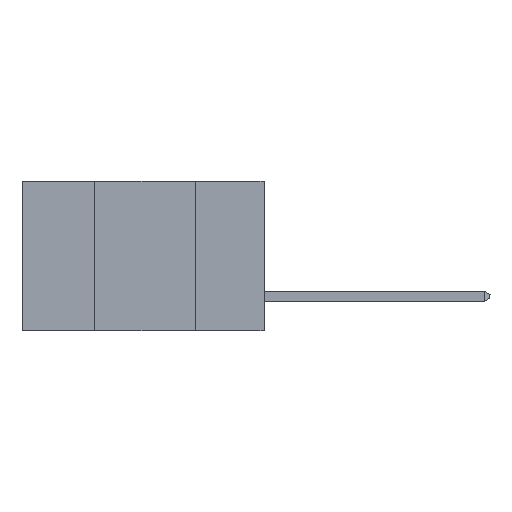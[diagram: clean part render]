
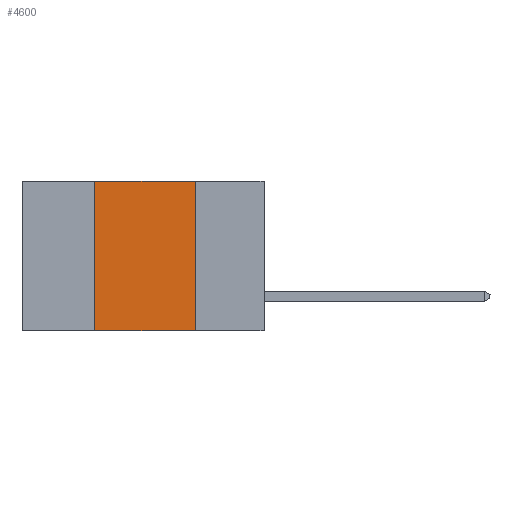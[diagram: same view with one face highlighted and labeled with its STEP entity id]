
A CAD part, left-side view. The second image highlights one B-rep face of the part: STEP entity #4600.
In plain terms, the highlighted planar face has unit normal (-1, 0, 0).
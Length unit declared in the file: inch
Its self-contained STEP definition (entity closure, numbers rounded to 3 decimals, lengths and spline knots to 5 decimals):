
#760 = VECTOR ( 'NONE', #7964, 39.37008 ) ;
#1302 = CARTESIAN_POINT ( 'NONE',  ( 0., 0.17, -0.37 ) ) ;
#1324 = ORIENTED_EDGE ( 'NONE', *, *, #4816, .F. ) ;
#1356 = CARTESIAN_POINT ( 'NONE',  ( 0., 0.6, 0. ) ) ;
#1605 = DIRECTION ( 'NONE',  ( 1., 0., 0. ) ) ;
#2115 = CARTESIAN_POINT ( 'NONE',  ( 0., 0.6, -0.37 ) ) ;
#2451 = LINE ( 'NONE', #1356, #6887 ) ;
#2771 = CARTESIAN_POINT ( 'NONE',  ( 0., 0.6, 0. ) ) ;
#3345 = VECTOR ( 'NONE', #13911, 39.37008 ) ;
#3355 = LINE ( 'NONE', #11182, #760 ) ;
#3362 = VERTEX_POINT ( 'NONE', #8556 ) ;
#3592 = PLANE ( 'NONE',  #10115 ) ;
#3668 = EDGE_CURVE ( 'NONE', #3362, #10784, #4863, .T. ) ;
#3770 = VERTEX_POINT ( 'NONE', #8732 ) ;
#4344 = EDGE_CURVE ( 'NONE', #6129, #10784, #7761, .T. ) ;
#4600 = ADVANCED_FACE ( 'NONE', ( #4975 ), #3592, .F. ) ;
#4816 = EDGE_CURVE ( 'NONE', #6129, #3770, #3355, .T. ) ;
#4863 = LINE ( 'NONE', #11534, #3345 ) ;
#4975 = FACE_OUTER_BOUND ( 'NONE', #6403, .T. ) ;
#5325 = ORIENTED_EDGE ( 'NONE', *, *, #3668, .F. ) ;
#6129 = VERTEX_POINT ( 'NONE', #7472 ) ;
#6403 = EDGE_LOOP ( 'NONE', ( #5325, #11475, #1324, #10087 ) ) ;
#6774 = EDGE_CURVE ( 'NONE', #3770, #3362, #2451, .T. ) ;
#6887 = VECTOR ( 'NONE', #13627, 39.37008 ) ;
#7472 = CARTESIAN_POINT ( 'NONE',  ( 0., 0.42, -0.37 ) ) ;
#7761 = LINE ( 'NONE', #2115, #8001 ) ;
#7964 = DIRECTION ( 'NONE',  ( 0., 0., 1. ) ) ;
#8001 = VECTOR ( 'NONE', #13445, 39.37008 ) ;
#8556 = CARTESIAN_POINT ( 'NONE',  ( 0., 0.17, 0. ) ) ;
#8732 = CARTESIAN_POINT ( 'NONE',  ( 0., 0.42, 0. ) ) ;
#10087 = ORIENTED_EDGE ( 'NONE', *, *, #4344, .T. ) ;
#10115 = AXIS2_PLACEMENT_3D ( 'NONE', #2771, #1605, #12685 ) ;
#10784 = VERTEX_POINT ( 'NONE', #1302 ) ;
#11182 = CARTESIAN_POINT ( 'NONE',  ( 0., 0.42, -0.37 ) ) ;
#11475 = ORIENTED_EDGE ( 'NONE', *, *, #6774, .F. ) ;
#11534 = CARTESIAN_POINT ( 'NONE',  ( 0., 0.17, -0.37 ) ) ;
#12685 = DIRECTION ( 'NONE',  ( 0., 0., -1. ) ) ;
#13445 = DIRECTION ( 'NONE',  ( 0., -1., 0. ) ) ;
#13627 = DIRECTION ( 'NONE',  ( 0., -1., 0. ) ) ;
#13911 = DIRECTION ( 'NONE',  ( 0., 0., -1. ) ) ;
